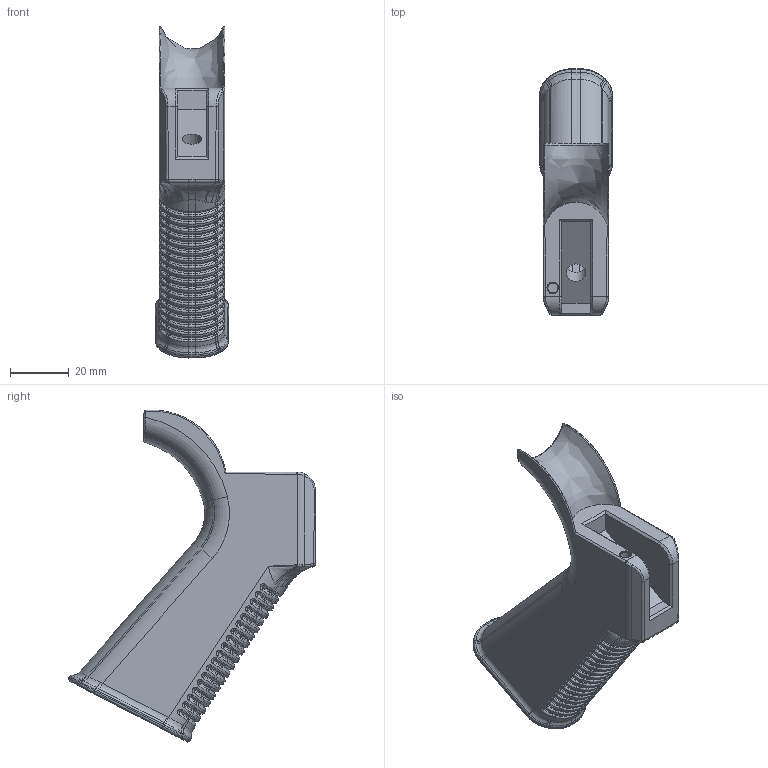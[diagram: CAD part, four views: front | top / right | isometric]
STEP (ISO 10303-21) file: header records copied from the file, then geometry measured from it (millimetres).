
FILE_DESCRIPTION(/* description */ (''),/* implementation_level */ '2;1');
FILE_NAME(/* name */ 'Ridged.step',/* time_stamp */ '2021-09-05T14:40:49-04:00',/* author */ (''),/* organization */ (''),/* preprocessor_version */ 'ST-DEVELOPER v18.1',/* originating_system */ 'Autodesk Translation Framework v10.10.0.1391',/* authorisation */ '');
FILE_SCHEMA (('AUTOMOTIVE_DESIGN { 1 0 10303 214 3 1 1 }'));
Products named in the file (1): Ridged
Bounding box: 24.83 x 83.89 x 112.88 mm (x, y, z)
Volume: 47357.7 mm3; surface area: 21134 mm2
Topology: 1 solids, 1 shells, 1100 faces, 2373 edges, 1272 vertices
Faces by surface type: bspline 488, cylinder 351, plane 164, torus 89, cone 8
Full cylindrical faces by diameter (mm): 3.4 x1, 6.8 x1, 14.521 x1, 16.771 x1
Entity records: 42132 total; most frequent: CARTESIAN_POINT 21054, ORIENTED_EDGE 4726, DIRECTION 3685, EDGE_CURVE 2363, AXIS2_PLACEMENT_3D 1475, VERTEX_POINT 1272, EDGE_LOOP 1109, FACE_OUTER_BOUND 1100
